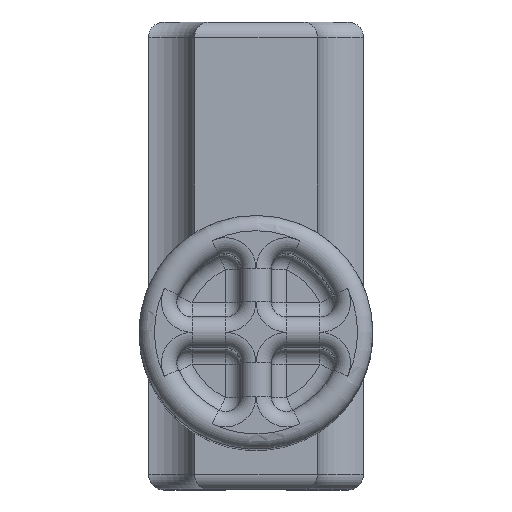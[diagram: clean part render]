
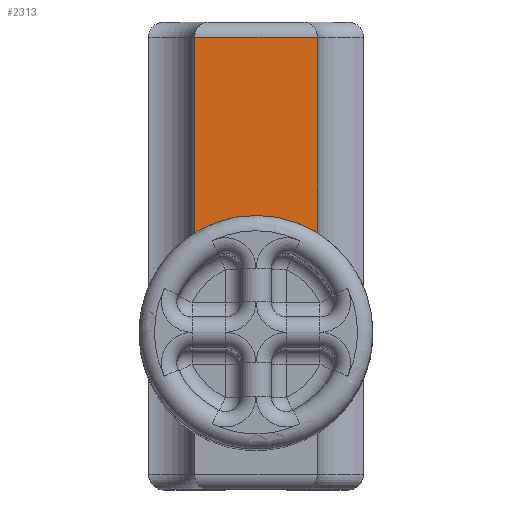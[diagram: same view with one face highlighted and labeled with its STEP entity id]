
A CAD part, top view. The second image highlights one B-rep face of the part: STEP entity #2313.
In plain terms, the highlighted planar face has unit normal (0, 0, 1).
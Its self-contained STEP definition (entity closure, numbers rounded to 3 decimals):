
#17 = DIRECTION ( 'NONE',  ( 0., 0., -1. ) ) ;
#125 = CARTESIAN_POINT ( 'NONE',  ( 10., -47.2, 17.5 ) ) ;
#256 = VERTEX_POINT ( 'NONE', #1766 ) ;
#259 = VERTEX_POINT ( 'NONE', #2472 ) ;
#311 = ORIENTED_EDGE ( 'NONE', *, *, #989, .T. ) ;
#343 = CARTESIAN_POINT ( 'NONE',  ( -10., 48.3, 17.5 ) ) ;
#520 = DIRECTION ( 'NONE',  ( -1., 0., 0. ) ) ;
#576 = EDGE_CURVE ( 'NONE', #2156, #259, #2087, .T. ) ;
#649 = DIRECTION ( 'NONE',  ( -1., 0., 0. ) ) ;
#717 = CARTESIAN_POINT ( 'NONE',  ( -10., 16.214, 17.5 ) ) ;
#747 = VERTEX_POINT ( 'NONE', #343 ) ;
#816 = DIRECTION ( 'NONE',  ( 0., 1., 0. ) ) ;
#832 = EDGE_LOOP ( 'NONE', ( #2095, #311, #1591, #838 ) ) ;
#838 = ORIENTED_EDGE ( 'NONE', *, *, #576, .T. ) ;
#989 = EDGE_CURVE ( 'NONE', #256, #747, #1298, .T. ) ;
#994 = CARTESIAN_POINT ( 'NONE',  ( -10., 48.3, 17.5 ) ) ;
#1107 = VECTOR ( 'NONE', #1110, 1000. ) ;
#1110 = DIRECTION ( 'NONE',  ( 0., -1., 0. ) ) ;
#1149 = VECTOR ( 'NONE', #520, 1000. ) ;
#1175 = LINE ( 'NONE', #2696, #1107 ) ;
#1298 = LINE ( 'NONE', #994, #1149 ) ;
#1345 = DIRECTION ( 'NONE',  ( 0., 0., -1. ) ) ;
#1400 = CARTESIAN_POINT ( 'NONE',  ( 0., 0., 17.5 ) ) ;
#1583 = AXIS2_PLACEMENT_3D ( 'NONE', #1400, #17, #1622 ) ;
#1591 = ORIENTED_EDGE ( 'NONE', *, *, #2297, .T. ) ;
#1622 = DIRECTION ( 'NONE',  ( -1., 0., 0. ) ) ;
#1766 = CARTESIAN_POINT ( 'NONE',  ( 10., 48.3, 17.5 ) ) ;
#1798 = CARTESIAN_POINT ( 'NONE',  ( 0., -25.4, 17.5 ) ) ;
#1918 = LINE ( 'NONE', #125, #2551 ) ;
#2032 = AXIS2_PLACEMENT_3D ( 'NONE', #1798, #1345, #649 ) ;
#2034 = PLANE ( 'NONE',  #2032 ) ;
#2087 = CIRCLE ( 'NONE', #1583, 19.05 ) ;
#2095 = ORIENTED_EDGE ( 'NONE', *, *, #2694, .T. ) ;
#2156 = VERTEX_POINT ( 'NONE', #717 ) ;
#2297 = EDGE_CURVE ( 'NONE', #747, #2156, #1175, .T. ) ;
#2313 = ADVANCED_FACE ( 'NONE', ( #2858 ), #2034, .F. ) ;
#2472 = CARTESIAN_POINT ( 'NONE',  ( 10., 16.214, 17.5 ) ) ;
#2551 = VECTOR ( 'NONE', #816, 1000. ) ;
#2694 = EDGE_CURVE ( 'NONE', #259, #256, #1918, .T. ) ;
#2696 = CARTESIAN_POINT ( 'NONE',  ( -10., -47.2, 17.5 ) ) ;
#2858 = FACE_OUTER_BOUND ( 'NONE', #832, .T. ) ;
